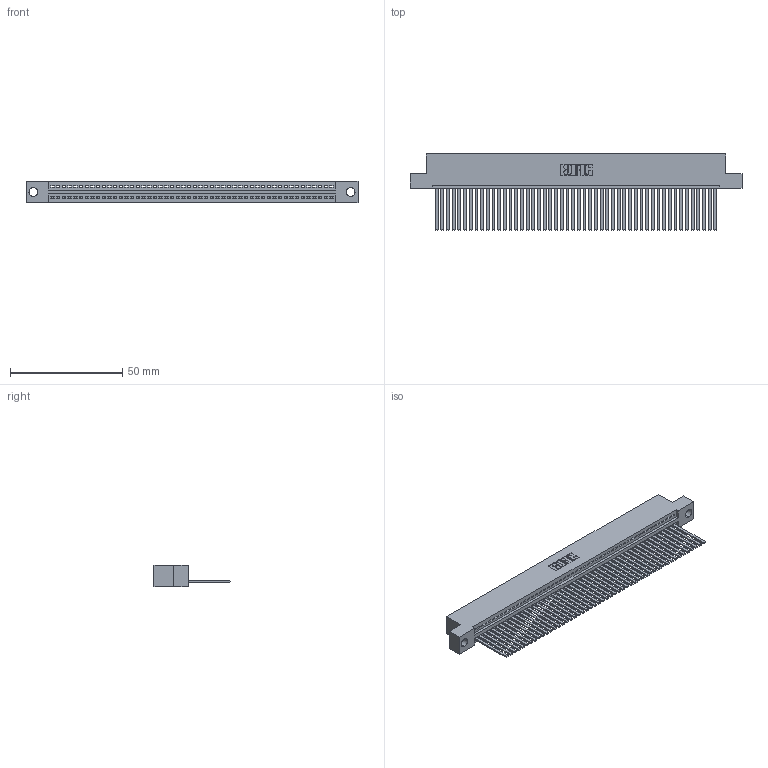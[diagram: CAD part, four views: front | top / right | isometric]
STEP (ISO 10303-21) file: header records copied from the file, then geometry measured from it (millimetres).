
FILE_DESCRIPTION (( 'STEP AP203' ), '1' );
FILE_NAME ('345-050-544-104.STEP', '2019-10-09T13:06:27', ( '' ), ( '' ), 'SwSTEP 2.0', 'SolidWorks 2016', '' );
FILE_SCHEMA (( 'CONFIG_CONTROL_DESIGN' ));
Length unit declared in the file: inch
Products named in the file (3): 345-292-001_345-293-144; 345 Part_Flush Mounting Lugs - 0.156 Dia-TH; 345-050-544-104
Assembly tree (51 placements, depth 2):
  345-050-544-104
    345 Part_Flush Mounting Lugs - 0.156 Dia-TH
    345-292-001_345-293-144  x50
Bounding box: 148.21 x 33.96 x 9.4 mm (x, y, z)
Volume: 14633.8 mm3; surface area: 21102.9 mm2
Topology: 51 solids, 51 shells, 2726 faces, 8241 edges, 5426 vertices
Faces by surface type: plane 1880, cylinder 846
Entity records: 36373 total; most frequent: CARTESIAN_POINT 6306, ORIENTED_EDGE 6290, DIRECTION 5493, EDGE_CURVE 3145, VECTOR 2817, LINE 2817, VERTEX_POINT 2094, AXIS2_PLACEMENT_3D 1338
